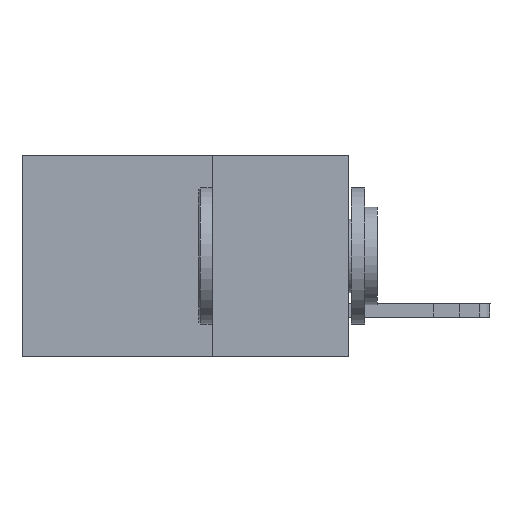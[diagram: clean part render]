
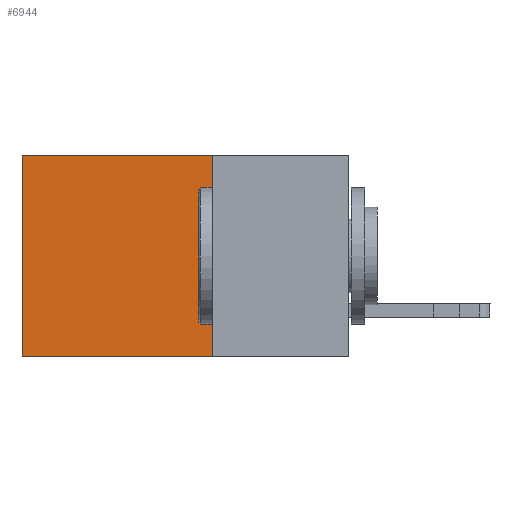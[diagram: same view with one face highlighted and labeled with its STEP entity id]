
A CAD part, left-side view. The second image highlights one B-rep face of the part: STEP entity #6944.
In plain terms, the highlighted planar face has unit normal (-1, 0, 0).
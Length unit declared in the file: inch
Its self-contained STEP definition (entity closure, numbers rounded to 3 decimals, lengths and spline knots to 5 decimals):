
#1 = CARTESIAN_POINT ( 'NONE',  ( 0.2615, 0.25, -0.37 ) ) ;
#50 = PLANE ( 'NONE',  #9247 ) ;
#176 = ORIENTED_EDGE ( 'NONE', *, *, #1318, .F. ) ;
#282 = CARTESIAN_POINT ( 'NONE',  ( 0.2615, 0.6, -0.37 ) ) ;
#634 = DIRECTION ( 'NONE',  ( 0., 0., -1. ) ) ;
#1318 = EDGE_CURVE ( 'NONE', #8096, #8418, #5177, .T. ) ;
#1886 = VERTEX_POINT ( 'NONE', #6363 ) ;
#1906 = CARTESIAN_POINT ( 'NONE',  ( 0.2615, 0.25, -0.37 ) ) ;
#2410 = VECTOR ( 'NONE', #5528, 39.37008 ) ;
#2708 = CARTESIAN_POINT ( 'NONE',  ( 0.2615, 0.6, 0. ) ) ;
#2873 = LINE ( 'NONE', #5469, #2410 ) ;
#2894 = ORIENTED_EDGE ( 'NONE', *, *, #10238, .F. ) ;
#3266 = EDGE_CURVE ( 'NONE', #1886, #6028, #10480, .T. ) ;
#4596 = EDGE_CURVE ( 'NONE', #6028, #8418, #2873, .T. ) ;
#5095 = DIRECTION ( 'NONE',  ( 0., 0., -1. ) ) ;
#5152 = CARTESIAN_POINT ( 'NONE',  ( 0.2615, 0.25, -0.37 ) ) ;
#5177 = LINE ( 'NONE', #1906, #7672 ) ;
#5235 = DIRECTION ( 'NONE',  ( 0., 1., 0. ) ) ;
#5469 = CARTESIAN_POINT ( 'NONE',  ( 0.2615, 0.6, -0.37 ) ) ;
#5528 = DIRECTION ( 'NONE',  ( 0., 0., -1. ) ) ;
#5645 = ORIENTED_EDGE ( 'NONE', *, *, #3266, .T. ) ;
#5664 = LINE ( 'NONE', #7364, #10784 ) ;
#6028 = VERTEX_POINT ( 'NONE', #2708 ) ;
#6363 = CARTESIAN_POINT ( 'NONE',  ( 0.2615, 0.25, 0. ) ) ;
#6632 = VECTOR ( 'NONE', #10372, 39.37008 ) ;
#6944 = ADVANCED_FACE ( 'NONE', ( #7572 ), #50, .F. ) ;
#7364 = CARTESIAN_POINT ( 'NONE',  ( 0.2615, 0.25, -0.37 ) ) ;
#7572 = FACE_OUTER_BOUND ( 'NONE', #9327, .T. ) ;
#7672 = VECTOR ( 'NONE', #5235, 39.37008 ) ;
#8035 = CARTESIAN_POINT ( 'NONE',  ( 0.2615, 0.25, 0. ) ) ;
#8096 = VERTEX_POINT ( 'NONE', #1 ) ;
#8118 = ORIENTED_EDGE ( 'NONE', *, *, #4596, .T. ) ;
#8418 = VERTEX_POINT ( 'NONE', #282 ) ;
#9247 = AXIS2_PLACEMENT_3D ( 'NONE', #5152, #10102, #5095 ) ;
#9327 = EDGE_LOOP ( 'NONE', ( #8118, #176, #2894, #5645 ) ) ;
#10102 = DIRECTION ( 'NONE',  ( 1., 0., 0. ) ) ;
#10238 = EDGE_CURVE ( 'NONE', #1886, #8096, #5664, .T. ) ;
#10372 = DIRECTION ( 'NONE',  ( 0., 1., 0. ) ) ;
#10480 = LINE ( 'NONE', #8035, #6632 ) ;
#10784 = VECTOR ( 'NONE', #634, 39.37008 ) ;
